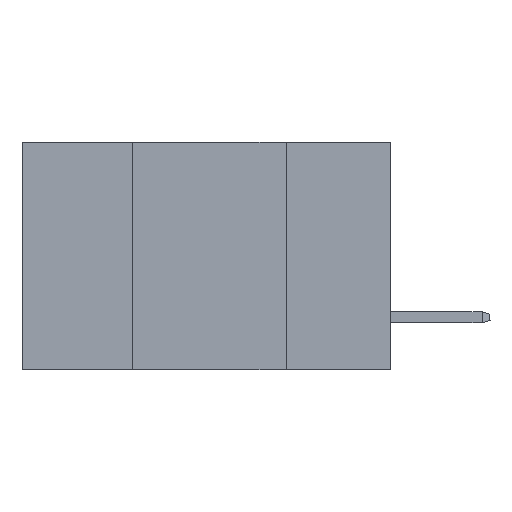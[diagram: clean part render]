
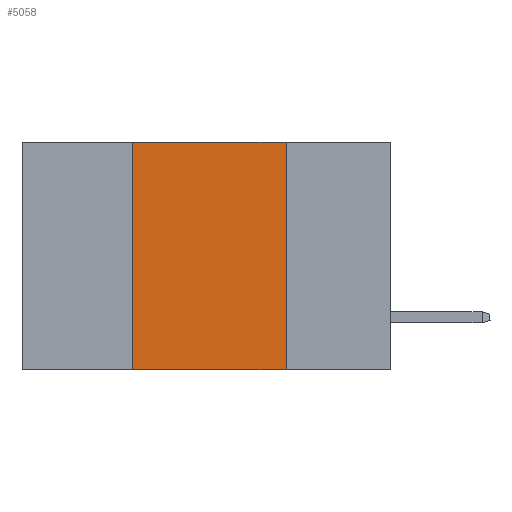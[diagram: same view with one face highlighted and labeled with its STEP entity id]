
A CAD part, left-side view. The second image highlights one B-rep face of the part: STEP entity #5058.
In plain terms, the highlighted planar face has unit normal (-1, 0, 0).
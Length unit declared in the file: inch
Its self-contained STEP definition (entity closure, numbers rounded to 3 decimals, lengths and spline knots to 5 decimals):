
#829 = AXIS2_PLACEMENT_3D ( 'NONE', #8055, #13933, #2423 ) ;
#1177 = LINE ( 'NONE', #9755, #8914 ) ;
#1263 = LINE ( 'NONE', #4333, #3558 ) ;
#1296 = CARTESIAN_POINT ( 'NONE',  ( 0., 0.17, 0. ) ) ;
#1655 = FACE_OUTER_BOUND ( 'NONE', #3746, .T. ) ;
#2048 = LINE ( 'NONE', #1296, #2939 ) ;
#2423 = DIRECTION ( 'NONE',  ( 0., 0., -1. ) ) ;
#2939 = VECTOR ( 'NONE', #7508, 39.37008 ) ;
#3558 = VECTOR ( 'NONE', #14548, 39.37008 ) ;
#3746 = EDGE_LOOP ( 'NONE', ( #14840, #13587, #4557, #4929 ) ) ;
#4233 = VERTEX_POINT ( 'NONE', #14364 ) ;
#4333 = CARTESIAN_POINT ( 'NONE',  ( 0., 0.6, -0.37 ) ) ;
#4557 = ORIENTED_EDGE ( 'NONE', *, *, #5062, .F. ) ;
#4929 = ORIENTED_EDGE ( 'NONE', *, *, #16876, .T. ) ;
#5058 = ADVANCED_FACE ( 'NONE', ( #1655 ), #16935, .F. ) ;
#5062 = EDGE_CURVE ( 'NONE', #4233, #11605, #1177, .T. ) ;
#6194 = VERTEX_POINT ( 'NONE', #16246 ) ;
#7508 = DIRECTION ( 'NONE',  ( 0., 0., -1. ) ) ;
#8055 = CARTESIAN_POINT ( 'NONE',  ( 0., 0.6, 0. ) ) ;
#8400 = DIRECTION ( 'NONE',  ( 0., -1., 0. ) ) ;
#8914 = VECTOR ( 'NONE', #11249, 39.37008 ) ;
#9091 = CARTESIAN_POINT ( 'NONE',  ( 0., 0.42, 0. ) ) ;
#9755 = CARTESIAN_POINT ( 'NONE',  ( 0., 0.42, 0. ) ) ;
#10337 = VERTEX_POINT ( 'NONE', #14448 ) ;
#10918 = EDGE_CURVE ( 'NONE', #6194, #10337, #2048, .T. ) ;
#11249 = DIRECTION ( 'NONE',  ( 0., 0., 1. ) ) ;
#11605 = VERTEX_POINT ( 'NONE', #9091 ) ;
#12231 = LINE ( 'NONE', #18421, #15640 ) ;
#13587 = ORIENTED_EDGE ( 'NONE', *, *, #17039, .F. ) ;
#13933 = DIRECTION ( 'NONE',  ( 1., 0., 0. ) ) ;
#14364 = CARTESIAN_POINT ( 'NONE',  ( 0., 0.42, -0.37 ) ) ;
#14448 = CARTESIAN_POINT ( 'NONE',  ( 0., 0.17, -0.37 ) ) ;
#14548 = DIRECTION ( 'NONE',  ( 0., -1., 0. ) ) ;
#14840 = ORIENTED_EDGE ( 'NONE', *, *, #10918, .F. ) ;
#15640 = VECTOR ( 'NONE', #8400, 39.37008 ) ;
#16246 = CARTESIAN_POINT ( 'NONE',  ( 0., 0.17, 0. ) ) ;
#16876 = EDGE_CURVE ( 'NONE', #4233, #10337, #1263, .T. ) ;
#16935 = PLANE ( 'NONE',  #829 ) ;
#17039 = EDGE_CURVE ( 'NONE', #11605, #6194, #12231, .T. ) ;
#18421 = CARTESIAN_POINT ( 'NONE',  ( 0., 0.6, 0. ) ) ;
